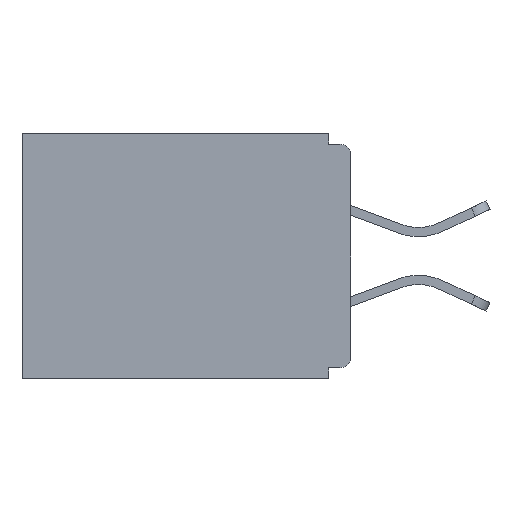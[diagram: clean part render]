
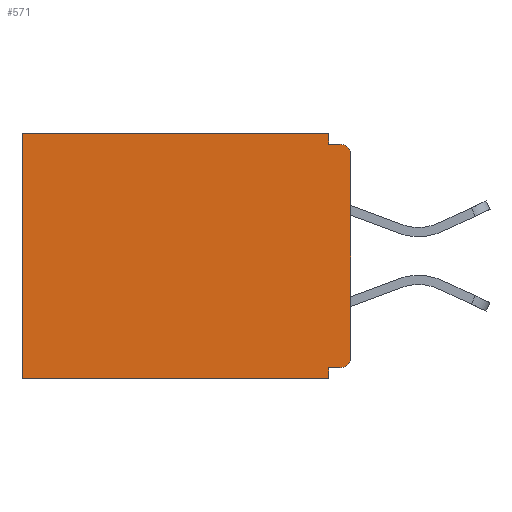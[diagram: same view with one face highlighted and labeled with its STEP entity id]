
A CAD part, left-side view. The second image highlights one B-rep face of the part: STEP entity #571.
In plain terms, the highlighted planar face has unit normal (-1, 0, 0).
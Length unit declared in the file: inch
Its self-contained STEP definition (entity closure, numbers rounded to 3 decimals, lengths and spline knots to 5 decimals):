
#295 = EDGE_CURVE ( 'NONE', #25431, #765, #7992, .T. ) ;
#545 = CARTESIAN_POINT ( 'NONE',  ( 0.298, 0.031, -0.343 ) ) ;
#571 = ADVANCED_FACE ( 'NONE', ( #14388 ), #15820, .F. ) ;
#765 = VERTEX_POINT ( 'NONE', #25585 ) ;
#809 = VERTEX_POINT ( 'NONE', #22804 ) ;
#891 = DIRECTION ( 'NONE',  ( 0., 0., -1. ) ) ;
#1586 = EDGE_CURVE ( 'NONE', #16994, #19102, #5047, .T. ) ;
#2147 = DIRECTION ( 'NONE',  ( 0., 1., 0. ) ) ;
#2630 = DIRECTION ( 'NONE',  ( 0., 0., -1. ) ) ;
#3332 = VECTOR ( 'NONE', #7865, 39.37008 ) ;
#3669 = EDGE_CURVE ( 'NONE', #809, #19102, #25680, .T. ) ;
#3998 = CARTESIAN_POINT ( 'NONE',  ( 0.298, 0.031, 0. ) ) ;
#4527 = VECTOR ( 'NONE', #6074, 39.37008 ) ;
#4666 = CARTESIAN_POINT ( 'NONE',  ( 0.298, 0.015, -0.313 ) ) ;
#5047 = CIRCLE ( 'NONE', #23667, 0.015 ) ;
#5271 = DIRECTION ( 'NONE',  ( 0., 0., -1. ) ) ;
#5520 = CARTESIAN_POINT ( 'NONE',  ( 0.298, 0.031, -0.343 ) ) ;
#5702 = CARTESIAN_POINT ( 'NONE',  ( 0.298, 0.46, -0.343 ) ) ;
#6074 = DIRECTION ( 'NONE',  ( 0., 1., 0. ) ) ;
#6754 = ORIENTED_EDGE ( 'NONE', *, *, #9300, .F. ) ;
#7025 = EDGE_LOOP ( 'NONE', ( #8902, #26508, #9167, #23438, #14361, #20950, #6754, #14921, #15254, #27410 ) ) ;
#7035 = LINE ( 'NONE', #27794, #4527 ) ;
#7068 = EDGE_CURVE ( 'NONE', #13565, #23587, #7035, .T. ) ;
#7284 = VECTOR ( 'NONE', #16094, 39.37008 ) ;
#7467 = CARTESIAN_POINT ( 'NONE',  ( 0.298, 0., 0. ) ) ;
#7865 = DIRECTION ( 'NONE',  ( 0., 0., -1. ) ) ;
#7992 = LINE ( 'NONE', #25641, #18151 ) ;
#8271 = CARTESIAN_POINT ( 'NONE',  ( 0.298, 0.031, -0.015 ) ) ;
#8439 = EDGE_CURVE ( 'NONE', #28126, #14396, #26514, .T. ) ;
#8576 = DIRECTION ( 'NONE',  ( 0., -1., 0. ) ) ;
#8902 = ORIENTED_EDGE ( 'NONE', *, *, #11006, .T. ) ;
#9167 = ORIENTED_EDGE ( 'NONE', *, *, #12168, .F. ) ;
#9199 = CARTESIAN_POINT ( 'NONE',  ( 0.298, 0.031, -0.328 ) ) ;
#9300 = EDGE_CURVE ( 'NONE', #12767, #13565, #22712, .T. ) ;
#9556 = AXIS2_PLACEMENT_3D ( 'NONE', #13897, #9567, #891 ) ;
#9567 = DIRECTION ( 'NONE',  ( -1., 0., 0. ) ) ;
#9679 = LINE ( 'NONE', #24642, #7284 ) ;
#11006 = EDGE_CURVE ( 'NONE', #809, #14396, #18575, .T. ) ;
#11844 = CARTESIAN_POINT ( 'NONE',  ( 0.298, 0.031, -0.343 ) ) ;
#12168 = EDGE_CURVE ( 'NONE', #25431, #28126, #27309, .T. ) ;
#12574 = CARTESIAN_POINT ( 'NONE',  ( 0.298, 0., -0.313 ) ) ;
#12683 = LINE ( 'NONE', #21625, #19817 ) ;
#12698 = EDGE_CURVE ( 'NONE', #16994, #12767, #12683, .T. ) ;
#12767 = VERTEX_POINT ( 'NONE', #9199 ) ;
#12806 = CARTESIAN_POINT ( 'NONE',  ( 0.298, 0.015, -0.015 ) ) ;
#13565 = VERTEX_POINT ( 'NONE', #5520 ) ;
#13897 = CARTESIAN_POINT ( 'NONE',  ( 0.298, 0.015, -0.03 ) ) ;
#14361 = ORIENTED_EDGE ( 'NONE', *, *, #27329, .T. ) ;
#14388 = FACE_OUTER_BOUND ( 'NONE', #7025, .T. ) ;
#14396 = VERTEX_POINT ( 'NONE', #12806 ) ;
#14819 = CARTESIAN_POINT ( 'NONE',  ( 0.298, 0., -0.015 ) ) ;
#14921 = ORIENTED_EDGE ( 'NONE', *, *, #12698, .F. ) ;
#15254 = ORIENTED_EDGE ( 'NONE', *, *, #1586, .T. ) ;
#15820 = PLANE ( 'NONE',  #18539 ) ;
#16094 = DIRECTION ( 'NONE',  ( 0., 0., -1. ) ) ;
#16994 = VERTEX_POINT ( 'NONE', #19190 ) ;
#18102 = DIRECTION ( 'NONE',  ( 0., 0., -1. ) ) ;
#18151 = VECTOR ( 'NONE', #19001, 39.37008 ) ;
#18539 = AXIS2_PLACEMENT_3D ( 'NONE', #24659, #22402, #18102 ) ;
#18575 = CIRCLE ( 'NONE', #9556, 0.015 ) ;
#19001 = DIRECTION ( 'NONE',  ( 0., 1., 0. ) ) ;
#19102 = VERTEX_POINT ( 'NONE', #12574 ) ;
#19190 = CARTESIAN_POINT ( 'NONE',  ( 0.298, 0.015, -0.328 ) ) ;
#19817 = VECTOR ( 'NONE', #2147, 39.37008 ) ;
#20760 = VECTOR ( 'NONE', #8576, 39.37008 ) ;
#20950 = ORIENTED_EDGE ( 'NONE', *, *, #7068, .F. ) ;
#21255 = VECTOR ( 'NONE', #5271, 39.37008 ) ;
#21625 = CARTESIAN_POINT ( 'NONE',  ( 0.298, 0., -0.328 ) ) ;
#22063 = DIRECTION ( 'NONE',  ( -1., 0., 0. ) ) ;
#22402 = DIRECTION ( 'NONE',  ( 1., 0., 0. ) ) ;
#22712 = LINE ( 'NONE', #11844, #3332 ) ;
#22804 = CARTESIAN_POINT ( 'NONE',  ( 0.298, 0., -0.03 ) ) ;
#23438 = ORIENTED_EDGE ( 'NONE', *, *, #295, .T. ) ;
#23587 = VERTEX_POINT ( 'NONE', #5702 ) ;
#23592 = VECTOR ( 'NONE', #2630, 39.37008 ) ;
#23667 = AXIS2_PLACEMENT_3D ( 'NONE', #4666, #22063, #24225 ) ;
#24225 = DIRECTION ( 'NONE',  ( 0., 0., -1. ) ) ;
#24642 = CARTESIAN_POINT ( 'NONE',  ( 0.298, 0.46, 0. ) ) ;
#24659 = CARTESIAN_POINT ( 'NONE',  ( 0.298, 0., 0. ) ) ;
#25431 = VERTEX_POINT ( 'NONE', #3998 ) ;
#25585 = CARTESIAN_POINT ( 'NONE',  ( 0.298, 0.46, 0. ) ) ;
#25641 = CARTESIAN_POINT ( 'NONE',  ( 0.298, 0., 0. ) ) ;
#25680 = LINE ( 'NONE', #7467, #21255 ) ;
#26508 = ORIENTED_EDGE ( 'NONE', *, *, #8439, .F. ) ;
#26514 = LINE ( 'NONE', #14819, #20760 ) ;
#27309 = LINE ( 'NONE', #545, #23592 ) ;
#27329 = EDGE_CURVE ( 'NONE', #765, #23587, #9679, .T. ) ;
#27410 = ORIENTED_EDGE ( 'NONE', *, *, #3669, .F. ) ;
#27794 = CARTESIAN_POINT ( 'NONE',  ( 0.298, 0., -0.343 ) ) ;
#28126 = VERTEX_POINT ( 'NONE', #8271 ) ;
